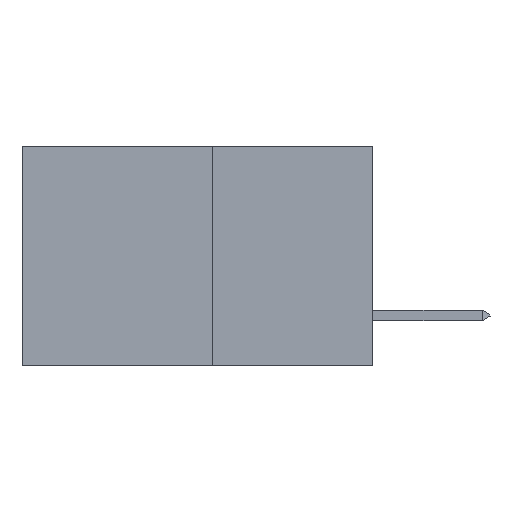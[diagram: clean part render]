
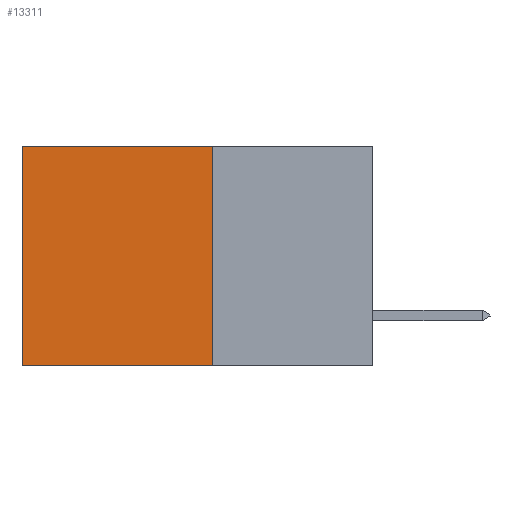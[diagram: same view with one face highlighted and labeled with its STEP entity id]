
A CAD part, left-side view. The second image highlights one B-rep face of the part: STEP entity #13311.
In plain terms, the highlighted planar face has unit normal (-1, 0, 0).
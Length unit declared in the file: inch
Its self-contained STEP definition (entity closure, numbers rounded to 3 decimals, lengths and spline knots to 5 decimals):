
#2024 = CARTESIAN_POINT ( 'NONE',  ( 0.277, 0.59, -0.37 ) ) ;
#2990 = DIRECTION ( 'NONE',  ( 0., 1., 0. ) ) ;
#3003 = CARTESIAN_POINT ( 'NONE',  ( 0.277, 0.59, -0.37 ) ) ;
#3873 = LINE ( 'NONE', #15313, #24304 ) ;
#4375 = CARTESIAN_POINT ( 'NONE',  ( 0.277, 0.27, -0.37 ) ) ;
#6166 = CARTESIAN_POINT ( 'NONE',  ( 0.277, 0.27, -0.37 ) ) ;
#6785 = PLANE ( 'NONE',  #21498 ) ;
#6888 = VERTEX_POINT ( 'NONE', #2024 ) ;
#6894 = VECTOR ( 'NONE', #2990, 39.37008 ) ;
#9518 = VECTOR ( 'NONE', #16620, 39.37008 ) ;
#9793 = ORIENTED_EDGE ( 'NONE', *, *, #14755, .F. ) ;
#9930 = VERTEX_POINT ( 'NONE', #27661 ) ;
#13311 = ADVANCED_FACE ( 'NONE', ( #19951 ), #6785, .F. ) ;
#13674 = LINE ( 'NONE', #18803, #6894 ) ;
#13950 = CARTESIAN_POINT ( 'NONE',  ( 0.277, 0.27, -0.37 ) ) ;
#14755 = EDGE_CURVE ( 'NONE', #18061, #6888, #3873, .T. ) ;
#15313 = CARTESIAN_POINT ( 'NONE',  ( 0.277, 0.27, -0.37 ) ) ;
#15754 = DIRECTION ( 'NONE',  ( 0., 1., 0. ) ) ;
#16390 = ORIENTED_EDGE ( 'NONE', *, *, #19661, .T. ) ;
#16620 = DIRECTION ( 'NONE',  ( 0., 0., -1. ) ) ;
#18061 = VERTEX_POINT ( 'NONE', #6166 ) ;
#18803 = CARTESIAN_POINT ( 'NONE',  ( 0.277, 0.27, 0. ) ) ;
#19661 = EDGE_CURVE ( 'NONE', #9930, #6888, #27787, .T. ) ;
#19870 = ORIENTED_EDGE ( 'NONE', *, *, #27260, .F. ) ;
#19951 = FACE_OUTER_BOUND ( 'NONE', #27860, .T. ) ;
#20820 = DIRECTION ( 'NONE',  ( 0., 0., -1. ) ) ;
#21015 = DIRECTION ( 'NONE',  ( 0., 0., -1. ) ) ;
#21118 = DIRECTION ( 'NONE',  ( 1., 0., 0. ) ) ;
#21162 = VECTOR ( 'NONE', #20820, 39.37008 ) ;
#21498 = AXIS2_PLACEMENT_3D ( 'NONE', #4375, #21118, #21015 ) ;
#22615 = LINE ( 'NONE', #13950, #21162 ) ;
#24304 = VECTOR ( 'NONE', #15754, 39.37008 ) ;
#24312 = VERTEX_POINT ( 'NONE', #29238 ) ;
#27260 = EDGE_CURVE ( 'NONE', #24312, #18061, #22615, .T. ) ;
#27380 = EDGE_CURVE ( 'NONE', #24312, #9930, #13674, .T. ) ;
#27661 = CARTESIAN_POINT ( 'NONE',  ( 0.277, 0.59, 0. ) ) ;
#27787 = LINE ( 'NONE', #3003, #9518 ) ;
#27860 = EDGE_LOOP ( 'NONE', ( #16390, #9793, #19870, #29284 ) ) ;
#29238 = CARTESIAN_POINT ( 'NONE',  ( 0.277, 0.27, 0. ) ) ;
#29284 = ORIENTED_EDGE ( 'NONE', *, *, #27380, .T. ) ;
